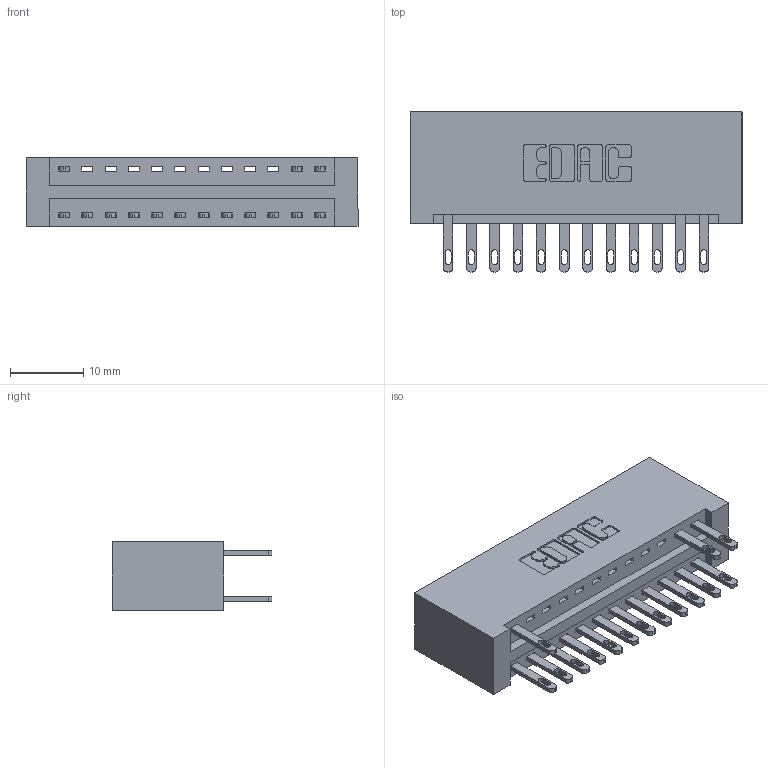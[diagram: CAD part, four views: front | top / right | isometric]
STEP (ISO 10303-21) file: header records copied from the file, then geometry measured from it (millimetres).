
FILE_DESCRIPTION (( 'STEP AP203' ), '1' );
FILE_NAME ('346-024-500-201.STEP', '2018-08-21T02:32:26', ( '' ), ( '' ), 'SwSTEP 2.0', 'SolidWorks 2016', '' );
FILE_SCHEMA (( 'CONFIG_CONTROL_DESIGN' ));
Length unit declared in the file: inch
Products named in the file (3): 346 Part_No Mounting Lugs; 345-292-001_345-293-100; 346-024-500-201
Assembly tree (16 placements, depth 2):
  346-024-500-201
    346 Part_No Mounting Lugs
    345-292-001_345-293-100  x15
Bounding box: 45.34 x 21.84 x 9.4 mm (x, y, z)
Volume: 4726.2 mm3; surface area: 5878.1 mm2
Topology: 16 solids, 16 shells, 888 faces, 2699 edges, 1798 vertices
Faces by surface type: plane 552, cylinder 336
Entity records: 11235 total; most frequent: CARTESIAN_POINT 1927, ORIENTED_EDGE 1870, DIRECTION 1737, EDGE_CURVE 935, VECTOR 759, LINE 759, VERTEX_POINT 622, AXIS2_PLACEMENT_3D 489
